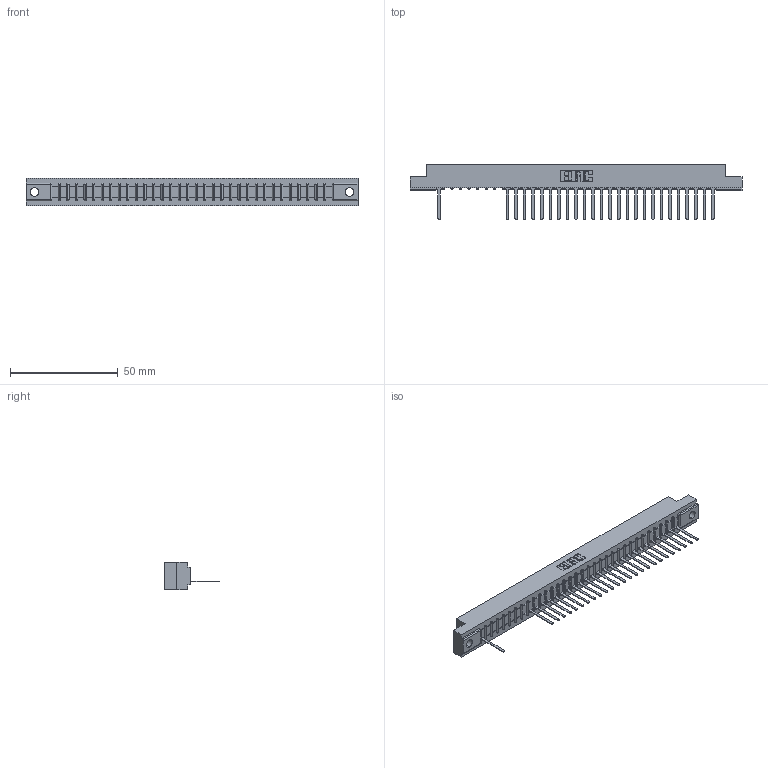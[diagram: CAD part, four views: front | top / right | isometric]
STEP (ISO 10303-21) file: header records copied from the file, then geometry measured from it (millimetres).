
FILE_DESCRIPTION (( 'STEP AP203' ), '1' );
FILE_NAME ('307-033-547-104.STEP', '2018-08-04T23:30:29', ( '' ), ( '' ), 'SwSTEP 2.0', 'SolidWorks 2016', '' );
FILE_SCHEMA (( 'CONFIG_CONTROL_DESIGN' ));
Length unit declared in the file: inch
Products named in the file (3): 307-033-547-104; 307 Part_.156 Dia Mounting Holes; 307-290-001_547
Assembly tree (27 placements, depth 2):
  307-033-547-104
    307 Part_.156 Dia Mounting Holes
    307-290-001_547  x26
Bounding box: 153.77 x 25.43 x 12.7 mm (x, y, z)
Volume: 15764.7 mm3; surface area: 16115.3 mm2
Topology: 27 solids, 27 shells, 1762 faces, 5019 edges, 3218 vertices
Faces by surface type: plane 1130, cylinder 564, sphere 68
Entity records: 29562 total; most frequent: CARTESIAN_POINT 5011, ORIENTED_EDGE 5002, DIRECTION 4863, EDGE_CURVE 2501, LINE 1923, VECTOR 1923, VERTEX_POINT 1618, AXIS2_PLACEMENT_3D 1470
